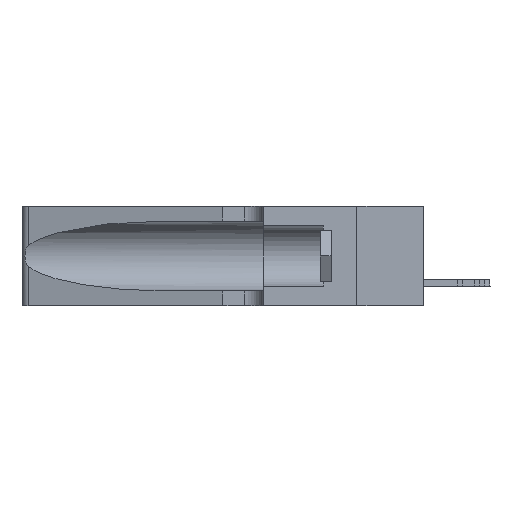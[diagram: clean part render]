
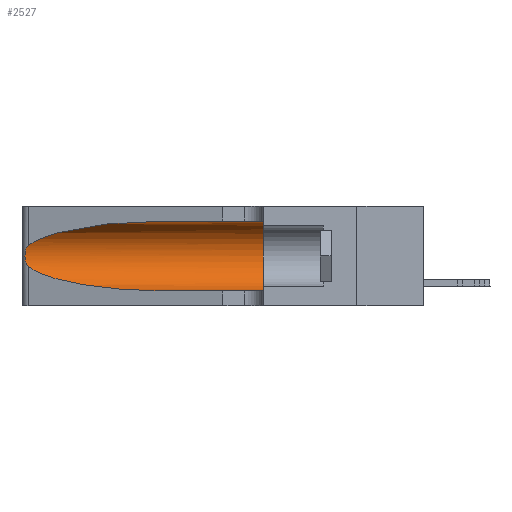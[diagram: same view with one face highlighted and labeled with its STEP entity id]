
A CAD part, left-side view. The second image highlights one B-rep face of the part: STEP entity #2527.
In plain terms, the highlighted cylindrical face has radius 3.308 mm (diameter 6.617 mm), a partial arc.
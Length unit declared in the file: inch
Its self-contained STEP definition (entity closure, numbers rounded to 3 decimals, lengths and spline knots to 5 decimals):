
#763 = CARTESIAN_POINT ( 'NONE',  ( 0.26075, 1.23896, 0.19203 ) ) ;
#967 = VERTEX_POINT ( 'NONE', #39995 ) ;
#1607 = DIRECTION ( 'NONE',  ( 0., 0., 1. ) ) ;
#1941 = ORIENTED_EDGE ( 'NONE', *, *, #42855, .T. ) ;
#2246 = LINE ( 'NONE', #22521, #2788 ) ;
#2527 = ADVANCED_FACE ( 'NONE', ( #12535 ), #44523, .F. ) ;
#2788 = VECTOR ( 'NONE', #5308, 39.37008 ) ;
#3184 = B_SPLINE_CURVE_WITH_KNOTS ( 'NONE', 3,
 ( #42191, #14310, #7820, #38886, #32075, #14740, #763, #11133, #28287, #39041, #18256, #34965, #10970, #18106 ),
 .UNSPECIFIED., .F., .F.,
 ( 4, 2, 2, 2, 2, 2, 4 ),
 ( 0., 0.00027, 0.00053, 0.00107, 0.0016, 0.00187, 0.00214 ),
 .UNSPECIFIED. ) ;
#5308 = DIRECTION ( 'NONE',  ( 0., -1., 0. ) ) ;
#6308 = CARTESIAN_POINT ( 'NONE',  ( 0.1305, 0.72297, 0.31525 ) ) ;
#7820 = CARTESIAN_POINT ( 'NONE',  ( 0.25639, 1.23184, 0.21858 ) ) ;
#8491 = CARTESIAN_POINT ( 'NONE',  ( 0.1305, 0.35, 0.185 ) ) ;
#8633 = DIRECTION ( 'NONE',  ( 0., 1., 0. ) ) ;
#8965 =( BOUNDED_CURVE ( )  B_SPLINE_CURVE ( 3, ( #42338, #11758, #38897, #25539 ),
 .UNSPECIFIED., .F., .T. ) 
 B_SPLINE_CURVE_WITH_KNOTS ( ( 4, 4 ),
 ( 1.5708, 2.84003 ),
 .UNSPECIFIED. ) 
 CURVE ( )  GEOMETRIC_REPRESENTATION_ITEM ( )  RATIONAL_B_SPLINE_CURVE ( ( 1., 0.87, 0.87, 1. ) ) 
 REPRESENTATION_ITEM ( '' )  );
#10726 = EDGE_CURVE ( 'NONE', #30766, #20789, #14382, .T. ) ;
#10970 = CARTESIAN_POINT ( 'NONE',  ( 0.25555, 1.22993, 0.14849 ) ) ;
#11133 = CARTESIAN_POINT ( 'NONE',  ( 0.26075, 1.23896, 0.178 ) ) ;
#11685 = DIRECTION ( 'NONE',  ( 0., -1., 0. ) ) ;
#11758 = CARTESIAN_POINT ( 'NONE',  ( 0.18966, 0.96281, 0.31525 ) ) ;
#12535 = FACE_OUTER_BOUND ( 'NONE', #17947, .T. ) ;
#12610 = EDGE_CURVE ( 'NONE', #26854, #967, #2246, .T. ) ;
#13811 = CARTESIAN_POINT ( 'NONE',  ( 0.1305, 0.72297, 0.05475 ) ) ;
#14116 = CARTESIAN_POINT ( 'NONE',  ( 0.1305, 0.72297, 0.05475 ) ) ;
#14310 = CARTESIAN_POINT ( 'NONE',  ( 0.25555, 1.22994, 0.2215 ) ) ;
#14382 = LINE ( 'NONE', #27796, #43156 ) ;
#14740 = CARTESIAN_POINT ( 'NONE',  ( 0.26018, 1.23835, 0.19895 ) ) ;
#14947 = CARTESIAN_POINT ( 'NONE',  ( 0.25487, 1.22718, 0.22369 ) ) ;
#17947 = EDGE_LOOP ( 'NONE', ( #1941, #37326, #40473, #38608, #35393, #35878 ) ) ;
#18106 = CARTESIAN_POINT ( 'NONE',  ( 0.25487, 1.22718, 0.14631 ) ) ;
#18150 = CARTESIAN_POINT ( 'NONE',  ( 0.25487, 1.22718, 0.14631 ) ) ;
#18256 = CARTESIAN_POINT ( 'NONE',  ( 0.25789, 1.23486, 0.15765 ) ) ;
#19271 = CIRCLE ( 'NONE', #39844, 0.13025 ) ;
#20789 = VERTEX_POINT ( 'NONE', #30614 ) ;
#22521 = CARTESIAN_POINT ( 'NONE',  ( 0.1305, 1.61858, 0.31525 ) ) ;
#22800 = VERTEX_POINT ( 'NONE', #18150 ) ;
#24251 = VERTEX_POINT ( 'NONE', #14947 ) ;
#24258 = EDGE_CURVE ( 'NONE', #967, #20789, #19271, .T. ) ;
#25539 = CARTESIAN_POINT ( 'NONE',  ( 0.25487, 1.22718, 0.22369 ) ) ;
#26854 = VERTEX_POINT ( 'NONE', #6308 ) ;
#27491 = CARTESIAN_POINT ( 'NONE',  ( 0.25487, 1.22718, 0.14631 ) ) ;
#27796 = CARTESIAN_POINT ( 'NONE',  ( 0.1305, 1.61858, 0.05475 ) ) ;
#28287 = CARTESIAN_POINT ( 'NONE',  ( 0.26017, 1.23833, 0.17102 ) ) ;
#29245 = AXIS2_PLACEMENT_3D ( 'NONE', #41287, #37965, #41418 ) ;
#30614 = CARTESIAN_POINT ( 'NONE',  ( 0.1305, 0.35, 0.05475 ) ) ;
#30766 = VERTEX_POINT ( 'NONE', #14116 ) ;
#31262 = CARTESIAN_POINT ( 'NONE',  ( 0.2373, 1.15595, 0.08982 ) ) ;
#32075 = CARTESIAN_POINT ( 'NONE',  ( 0.25854, 1.2359, 0.20912 ) ) ;
#32796 = EDGE_CURVE ( 'NONE', #22800, #30766, #44758, .T. ) ;
#34605 = CARTESIAN_POINT ( 'NONE',  ( 0.18966, 0.96281, 0.05475 ) ) ;
#34965 = CARTESIAN_POINT ( 'NONE',  ( 0.25639, 1.23186, 0.15144 ) ) ;
#35393 = ORIENTED_EDGE ( 'NONE', *, *, #24258, .F. ) ;
#35878 = ORIENTED_EDGE ( 'NONE', *, *, #12610, .F. ) ;
#37326 = ORIENTED_EDGE ( 'NONE', *, *, #40971, .T. ) ;
#37965 = DIRECTION ( 'NONE',  ( 0., -1., 0. ) ) ;
#38608 = ORIENTED_EDGE ( 'NONE', *, *, #10726, .T. ) ;
#38886 = CARTESIAN_POINT ( 'NONE',  ( 0.25787, 1.23484, 0.2124 ) ) ;
#38897 = CARTESIAN_POINT ( 'NONE',  ( 0.2373, 1.15595, 0.28018 ) ) ;
#39041 = CARTESIAN_POINT ( 'NONE',  ( 0.25856, 1.23593, 0.16098 ) ) ;
#39844 = AXIS2_PLACEMENT_3D ( 'NONE', #8491, #8633, #1607 ) ;
#39995 = CARTESIAN_POINT ( 'NONE',  ( 0.1305, 0.35, 0.31525 ) ) ;
#40473 = ORIENTED_EDGE ( 'NONE', *, *, #32796, .T. ) ;
#40971 = EDGE_CURVE ( 'NONE', #24251, #22800, #3184, .T. ) ;
#41287 = CARTESIAN_POINT ( 'NONE',  ( 0.1305, 1.61858, 0.185 ) ) ;
#41418 = DIRECTION ( 'NONE',  ( 0., 0., -1. ) ) ;
#42191 = CARTESIAN_POINT ( 'NONE',  ( 0.25487, 1.22718, 0.22369 ) ) ;
#42338 = CARTESIAN_POINT ( 'NONE',  ( 0.1305, 0.72297, 0.31525 ) ) ;
#42855 = EDGE_CURVE ( 'NONE', #26854, #24251, #8965, .T. ) ;
#43156 = VECTOR ( 'NONE', #11685, 39.37008 ) ;
#44523 = CYLINDRICAL_SURFACE ( 'NONE', #29245, 0.13025 ) ;
#44758 =( BOUNDED_CURVE ( )  B_SPLINE_CURVE ( 3, ( #27491, #31262, #34605, #13811 ),
 .UNSPECIFIED., .F., .T. ) 
 B_SPLINE_CURVE_WITH_KNOTS ( ( 4, 4 ),
 ( 3.44316, 4.71239 ),
 .UNSPECIFIED. ) 
 CURVE ( )  GEOMETRIC_REPRESENTATION_ITEM ( )  RATIONAL_B_SPLINE_CURVE ( ( 1., 0.87, 0.87, 1. ) ) 
 REPRESENTATION_ITEM ( '' )  );
